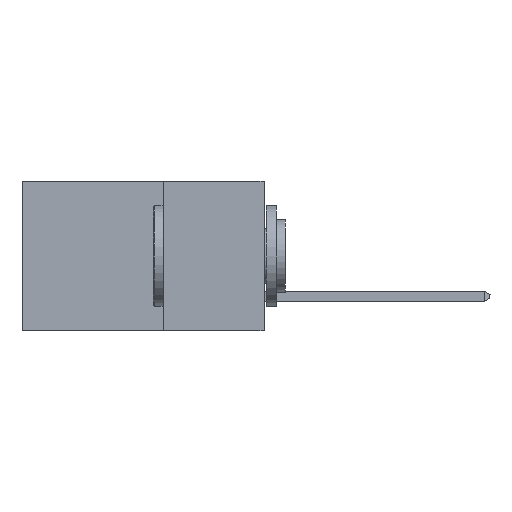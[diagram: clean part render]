
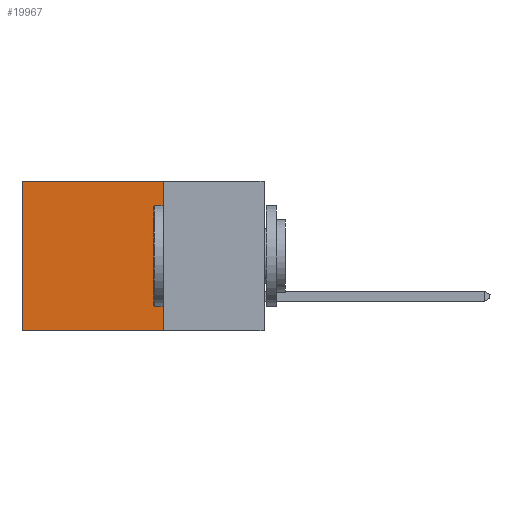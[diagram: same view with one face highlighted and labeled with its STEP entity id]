
A CAD part, left-side view. The second image highlights one B-rep face of the part: STEP entity #19967.
In plain terms, the highlighted planar face has unit normal (-1, 0, 0).
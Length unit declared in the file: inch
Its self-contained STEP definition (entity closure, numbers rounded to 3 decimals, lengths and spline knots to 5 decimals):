
#672 = ORIENTED_EDGE ( 'NONE', *, *, #3338, .F. ) ;
#3137 = CARTESIAN_POINT ( 'NONE',  ( 0.2615, 0.25, -0.37 ) ) ;
#3338 = EDGE_CURVE ( 'NONE', #19398, #6477, #14380, .T. ) ;
#3813 = VERTEX_POINT ( 'NONE', #16529 ) ;
#4399 = CARTESIAN_POINT ( 'NONE',  ( 0.2615, 0.25, 0. ) ) ;
#5693 = CARTESIAN_POINT ( 'NONE',  ( 0.2615, 0.25, -0.37 ) ) ;
#5714 = LINE ( 'NONE', #4399, #11676 ) ;
#6477 = VERTEX_POINT ( 'NONE', #8662 ) ;
#7959 = DIRECTION ( 'NONE',  ( 0., 1., 0. ) ) ;
#8143 = LINE ( 'NONE', #21302, #11955 ) ;
#8449 = VECTOR ( 'NONE', #7959, 39.37008 ) ;
#8585 = DIRECTION ( 'NONE',  ( 0., 0., -1. ) ) ;
#8641 = EDGE_CURVE ( 'NONE', #9727, #6477, #8143, .T. ) ;
#8662 = CARTESIAN_POINT ( 'NONE',  ( 0.2615, 0.6, -0.37 ) ) ;
#9727 = VERTEX_POINT ( 'NONE', #16770 ) ;
#10140 = ORIENTED_EDGE ( 'NONE', *, *, #10289, .F. ) ;
#10289 = EDGE_CURVE ( 'NONE', #3813, #19398, #18814, .T. ) ;
#10862 = EDGE_CURVE ( 'NONE', #3813, #9727, #5714, .T. ) ;
#11676 = VECTOR ( 'NONE', #19007, 39.37008 ) ;
#11955 = VECTOR ( 'NONE', #19691, 39.37008 ) ;
#12794 = ORIENTED_EDGE ( 'NONE', *, *, #8641, .T. ) ;
#13697 = CARTESIAN_POINT ( 'NONE',  ( 0.2615, 0.25, -0.37 ) ) ;
#14380 = LINE ( 'NONE', #3137, #8449 ) ;
#14381 = FACE_OUTER_BOUND ( 'NONE', #19362, .T. ) ;
#14494 = DIRECTION ( 'NONE',  ( 1., 0., 0. ) ) ;
#15096 = ORIENTED_EDGE ( 'NONE', *, *, #10862, .T. ) ;
#15486 = VECTOR ( 'NONE', #8585, 39.37008 ) ;
#16346 = CARTESIAN_POINT ( 'NONE',  ( 0.2615, 0.25, -0.37 ) ) ;
#16529 = CARTESIAN_POINT ( 'NONE',  ( 0.2615, 0.25, 0. ) ) ;
#16770 = CARTESIAN_POINT ( 'NONE',  ( 0.2615, 0.6, 0. ) ) ;
#18814 = LINE ( 'NONE', #13697, #15486 ) ;
#19007 = DIRECTION ( 'NONE',  ( 0., 1., 0. ) ) ;
#19362 = EDGE_LOOP ( 'NONE', ( #12794, #672, #10140, #15096 ) ) ;
#19375 = AXIS2_PLACEMENT_3D ( 'NONE', #16346, #14494, #21129 ) ;
#19398 = VERTEX_POINT ( 'NONE', #5693 ) ;
#19691 = DIRECTION ( 'NONE',  ( 0., 0., -1. ) ) ;
#19967 = ADVANCED_FACE ( 'NONE', ( #14381 ), #21020, .F. ) ;
#21020 = PLANE ( 'NONE',  #19375 ) ;
#21129 = DIRECTION ( 'NONE',  ( 0., 0., -1. ) ) ;
#21302 = CARTESIAN_POINT ( 'NONE',  ( 0.2615, 0.6, -0.37 ) ) ;
